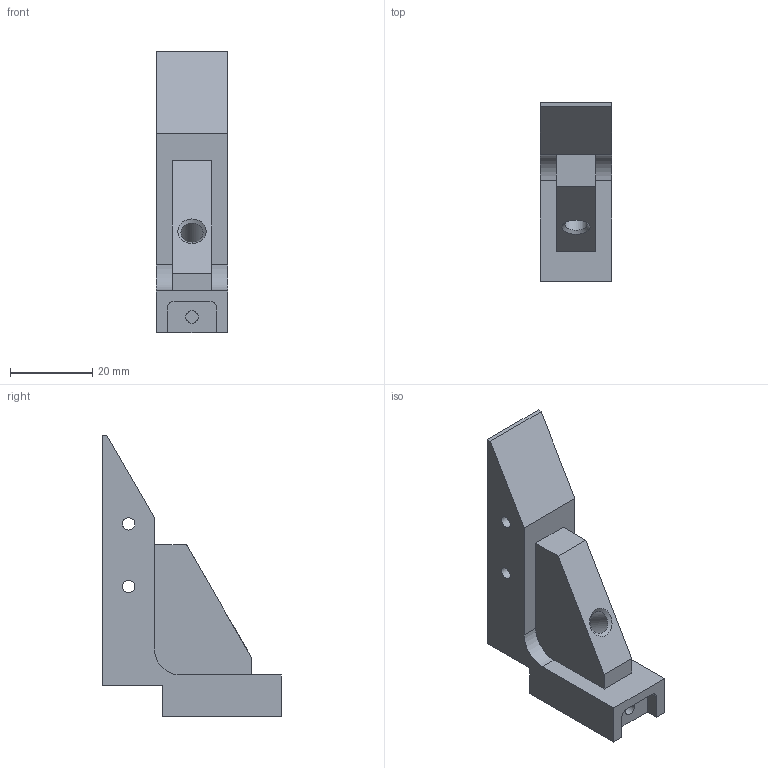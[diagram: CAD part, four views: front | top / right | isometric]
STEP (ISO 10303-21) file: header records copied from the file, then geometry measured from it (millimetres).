
FILE_DESCRIPTION (( 'STEP AP214' ), '1' );
FILE_NAME ('No_Safety_Reinforced_Grip_Part.step', '2016-01-30T20:06:12', ( 'WarFairy' ), ( '' ), 'SwSTEP 2.0', 'SolidWorks 2015', '' );
FILE_SCHEMA (( 'AUTOMOTIVE_DESIGN' ));
Length unit declared in the file: millimetre
Products named in the file (1): No_Safety_Reinforced_Grip_Part
Bounding box: 17.53 x 43.56 x 68.58 mm (x, y, z)
Volume: 18321.1 mm3; surface area: 8144.3 mm2
Topology: 1 solids, 1 shells, 53 faces, 148 edges, 99 vertices
Faces by surface type: plane 41, cylinder 11, cone 1
Full cylindrical faces by diameter (mm): 3 x5, 5.41 x1
Entity records: 1700 total; most frequent: CARTESIAN_POINT 296, ORIENTED_EDGE 278, DIRECTION 268, EDGE_CURVE 139, LINE 116, VECTOR 116, VERTEX_POINT 97, AXIS2_PLACEMENT_3D 76
